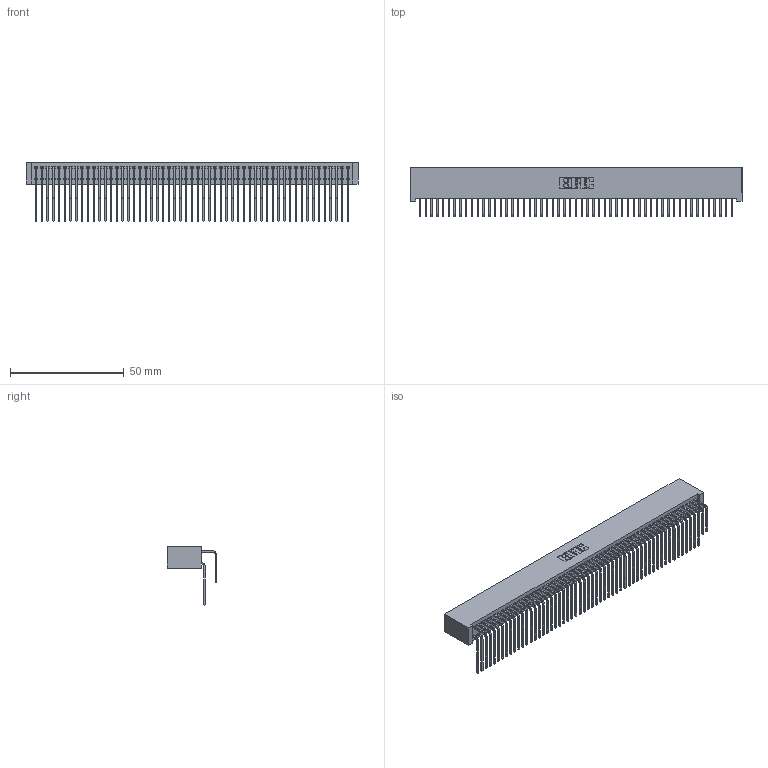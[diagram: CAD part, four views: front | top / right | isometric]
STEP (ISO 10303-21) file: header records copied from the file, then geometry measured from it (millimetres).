
FILE_DESCRIPTION (( 'STEP AP203' ), '1' );
FILE_NAME ('392-110-558-201.STEP', '2018-08-18T22:01:31', ( '' ), ( '' ), 'SwSTEP 2.0', 'SolidWorks 2016', '' );
FILE_SCHEMA (( 'CONFIG_CONTROL_DESIGN' ));
Length unit declared in the file: inch
Products named in the file (4): 345-292-001_558 Tail - 2; 392-110-558-201; 342 Part_Lugless; 345-292-001_558 559 Tail - 1
Assembly tree (111 placements, depth 2):
  392-110-558-201
    342 Part_Lugless
    345-292-001_558 559 Tail - 1  x55
    345-292-001_558 Tail - 2  x55
Bounding box: 145.95 x 21.91 x 25.78 mm (x, y, z)
Volume: 14249 mm3; surface area: 26831 mm2
Topology: 111 solids, 111 shells, 6042 faces, 17985 edges, 11842 vertices
Faces by surface type: plane 4242, cylinder 1800
Entity records: 35077 total; most frequent: CARTESIAN_POINT 5845, ORIENTED_EDGE 5730, DIRECTION 4945, EDGE_CURVE 2865, VECTOR 2705, LINE 2705, VERTEX_POINT 1906, AXIS2_PLACEMENT_3D 1120
